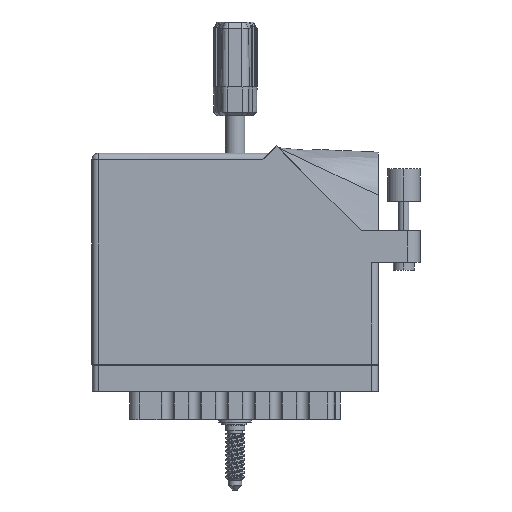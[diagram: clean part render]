
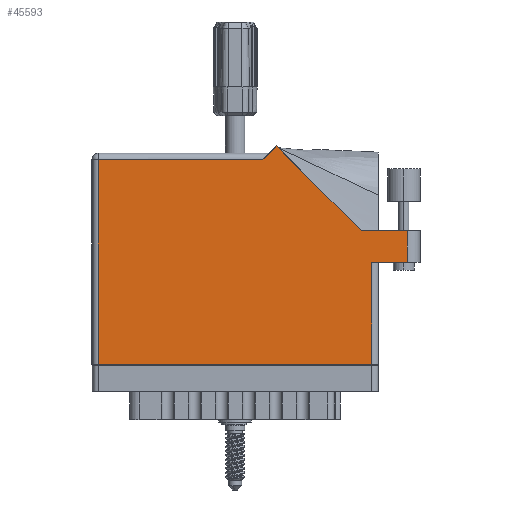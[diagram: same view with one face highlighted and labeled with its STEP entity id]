
A CAD part, front view. The second image highlights one B-rep face of the part: STEP entity #45593.
In plain terms, the highlighted face is planar.
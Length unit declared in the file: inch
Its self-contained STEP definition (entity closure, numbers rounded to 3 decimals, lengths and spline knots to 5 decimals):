
#1956 = VERTEX_POINT ( 'NONE', #47557 ) ;
#2844 = ORIENTED_EDGE ( 'NONE', *, *, #12818, .T. ) ;
#3514 = DIRECTION ( 'NONE',  ( 0., -1., 0. ) ) ;
#4139 = VERTEX_POINT ( 'NONE', #34296 ) ;
#4157 = VERTEX_POINT ( 'NONE', #18292 ) ;
#7144 = DIRECTION ( 'NONE',  ( -1., 0., 0. ) ) ;
#7292 = LINE ( 'NONE', #11768, #49457 ) ;
#11768 = CARTESIAN_POINT ( 'NONE',  ( 0., 1.968, 0. ) ) ;
#11941 = VERTEX_POINT ( 'NONE', #56797 ) ;
#12341 = ORIENTED_EDGE ( 'NONE', *, *, #69899, .T. ) ;
#12818 = EDGE_CURVE ( 'NONE', #46225, #1956, #57941, .T. ) ;
#13375 = VERTEX_POINT ( 'NONE', #55372 ) ;
#13540 = CARTESIAN_POINT ( 'NONE',  ( 2.693, 0.98, 0. ) ) ;
#14924 = LINE ( 'NONE', #13540, #59652 ) ;
#15313 = CARTESIAN_POINT ( 'NONE',  ( 1.705, 2.03, 0. ) ) ;
#17137 = LINE ( 'NONE', #29971, #66807 ) ;
#17496 = VECTOR ( 'NONE', #32378, 39.37008 ) ;
#18292 = CARTESIAN_POINT ( 'NONE',  ( 3.03, 0.98, 0. ) ) ;
#19359 = EDGE_CURVE ( 'NONE', #13375, #4157, #82276, .T. ) ;
#22076 = DIRECTION ( 'NONE',  ( 1., 0., 0. ) ) ;
#22520 = EDGE_CURVE ( 'NONE', #11941, #70856, #17137, .T. ) ;
#22715 = CARTESIAN_POINT ( 'NONE',  ( 3.03, 1.287, 0. ) ) ;
#22803 = CARTESIAN_POINT ( 'NONE',  ( 0., 2.03, 0. ) ) ;
#22991 = AXIS2_PLACEMENT_3D ( 'NONE', #22803, #46686, #7144 ) ;
#23448 = VECTOR ( 'NONE', #31944, 39.37008 ) ;
#29276 = DIRECTION ( 'NONE',  ( -0.707, 0.707, 0. ) ) ;
#29971 = CARTESIAN_POINT ( 'NONE',  ( 2.58942, 1.287, 0. ) ) ;
#31944 = DIRECTION ( 'NONE',  ( -0.707, -0.707, 0. ) ) ;
#32378 = DIRECTION ( 'NONE',  ( -1., 0., 0. ) ) ;
#32570 = VECTOR ( 'NONE', #52185, 39.37008 ) ;
#34296 = CARTESIAN_POINT ( 'NONE',  ( 3.03, 1.287, 0. ) ) ;
#35921 = CARTESIAN_POINT ( 'NONE',  ( 2.755, 0.98, 0. ) ) ;
#37334 = CARTESIAN_POINT ( 'NONE',  ( 0., 0., 0. ) ) ;
#38609 = VECTOR ( 'NONE', #86894, 39.37008 ) ;
#42210 = VERTEX_POINT ( 'NONE', #66638 ) ;
#44481 = LINE ( 'NONE', #15313, #23448 ) ;
#45593 = ADVANCED_FACE ( 'NONE', ( #55037 ), #70342, .F. ) ;
#46225 = VERTEX_POINT ( 'NONE', #68957 ) ;
#46686 = DIRECTION ( 'NONE',  ( 0., 0., -1. ) ) ;
#46790 = EDGE_CURVE ( 'NONE', #4157, #4139, #83362, .T. ) ;
#46927 = EDGE_CURVE ( 'NONE', #4139, #11941, #70897, .T. ) ;
#47557 = CARTESIAN_POINT ( 'NONE',  ( 0.062, 0., 0. ) ) ;
#47795 = ORIENTED_EDGE ( 'NONE', *, *, #84082, .T. ) ;
#48995 = LINE ( 'NONE', #37334, #56519 ) ;
#49457 = VECTOR ( 'NONE', #66249, 39.37008 ) ;
#51294 = ORIENTED_EDGE ( 'NONE', *, *, #22520, .T. ) ;
#52185 = DIRECTION ( 'NONE',  ( 1., 0., 0. ) ) ;
#53965 = ORIENTED_EDGE ( 'NONE', *, *, #19359, .T. ) ;
#54442 = ORIENTED_EDGE ( 'NONE', *, *, #89403, .T. ) ;
#55037 = FACE_OUTER_BOUND ( 'NONE', #55244, .T. ) ;
#55244 = EDGE_LOOP ( 'NONE', ( #53965, #76214, #85218, #51294, #12341, #47795, #2844, #61302, #54442 ) ) ;
#55372 = CARTESIAN_POINT ( 'NONE',  ( 2.693, 0.98, 0. ) ) ;
#56519 = VECTOR ( 'NONE', #22076, 39.37008 ) ;
#56704 = EDGE_CURVE ( 'NONE', #1956, #42210, #48995, .T. ) ;
#56797 = CARTESIAN_POINT ( 'NONE',  ( 2.58942, 1.287, 0. ) ) ;
#57941 = LINE ( 'NONE', #75098, #92711 ) ;
#59652 = VECTOR ( 'NONE', #76423, 39.37008 ) ;
#61302 = ORIENTED_EDGE ( 'NONE', *, *, #56704, .T. ) ;
#66249 = DIRECTION ( 'NONE',  ( -1., 0., 0. ) ) ;
#66638 = CARTESIAN_POINT ( 'NONE',  ( 2.693, 0., 0. ) ) ;
#66807 = VECTOR ( 'NONE', #29276, 39.37008 ) ;
#68957 = CARTESIAN_POINT ( 'NONE',  ( 0.062, 1.968, 0. ) ) ;
#69899 = EDGE_CURVE ( 'NONE', #70856, #88671, #44481, .T. ) ;
#70342 = PLANE ( 'NONE',  #22991 ) ;
#70856 = VERTEX_POINT ( 'NONE', #101454 ) ;
#70897 = LINE ( 'NONE', #79606, #17496 ) ;
#75098 = CARTESIAN_POINT ( 'NONE',  ( 0.062, 0., 0. ) ) ;
#75301 = CARTESIAN_POINT ( 'NONE',  ( 1.643, 1.968, 0. ) ) ;
#76214 = ORIENTED_EDGE ( 'NONE', *, *, #46790, .T. ) ;
#76423 = DIRECTION ( 'NONE',  ( 0., 1., 0. ) ) ;
#79606 = CARTESIAN_POINT ( 'NONE',  ( 3.155, 1.287, 0. ) ) ;
#82276 = LINE ( 'NONE', #35921, #32570 ) ;
#83362 = LINE ( 'NONE', #22715, #38609 ) ;
#84082 = EDGE_CURVE ( 'NONE', #88671, #46225, #7292, .T. ) ;
#85218 = ORIENTED_EDGE ( 'NONE', *, *, #46927, .T. ) ;
#86894 = DIRECTION ( 'NONE',  ( 0., 1., 0. ) ) ;
#88671 = VERTEX_POINT ( 'NONE', #75301 ) ;
#89403 = EDGE_CURVE ( 'NONE', #42210, #13375, #14924, .T. ) ;
#92711 = VECTOR ( 'NONE', #3514, 39.37008 ) ;
#101454 = CARTESIAN_POINT ( 'NONE',  ( 1.77571, 2.10071, 0. ) ) ;
